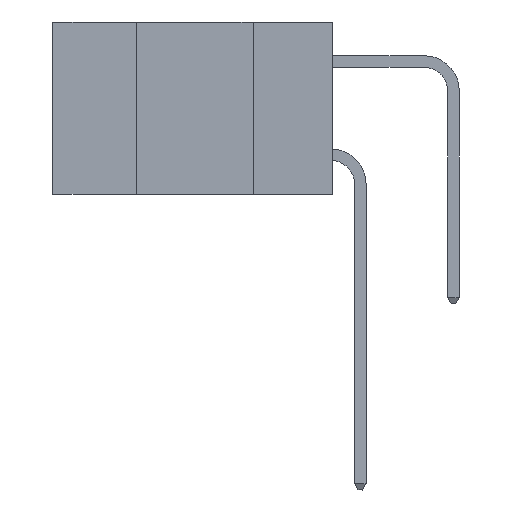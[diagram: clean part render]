
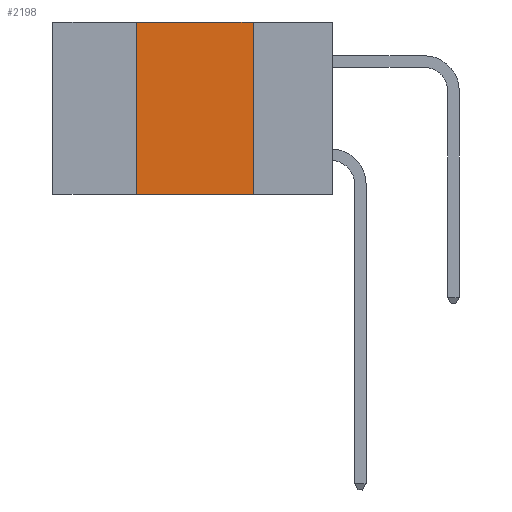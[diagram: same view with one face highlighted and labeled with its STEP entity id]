
A CAD part, left-side view. The second image highlights one B-rep face of the part: STEP entity #2198.
In plain terms, the highlighted planar face has unit normal (-1, 0, 0).
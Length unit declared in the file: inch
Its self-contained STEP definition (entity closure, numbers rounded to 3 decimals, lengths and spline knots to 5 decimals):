
#159 = CARTESIAN_POINT ( 'NONE',  ( 0., 0.17, 0. ) ) ;
#557 = VERTEX_POINT ( 'NONE', #20466 ) ;
#759 = VECTOR ( 'NONE', #14729, 39.37008 ) ;
#1258 = CARTESIAN_POINT ( 'NONE',  ( 0., 0.42, -0.37 ) ) ;
#1286 = LINE ( 'NONE', #1750, #15073 ) ;
#1750 = CARTESIAN_POINT ( 'NONE',  ( 0., 0.6, 0. ) ) ;
#1752 = LINE ( 'NONE', #10698, #31308 ) ;
#1899 = PLANE ( 'NONE',  #5361 ) ;
#1996 = VERTEX_POINT ( 'NONE', #25617 ) ;
#2198 = ADVANCED_FACE ( 'NONE', ( #20669 ), #1899, .F. ) ;
#3216 = DIRECTION ( 'NONE',  ( 0., -1., 0. ) ) ;
#5361 = AXIS2_PLACEMENT_3D ( 'NONE', #18979, #14195, #6666 ) ;
#6666 = DIRECTION ( 'NONE',  ( 0., 0., -1. ) ) ;
#7816 = EDGE_CURVE ( 'NONE', #21736, #1996, #13794, .T. ) ;
#10005 = DIRECTION ( 'NONE',  ( 0., 0., -1. ) ) ;
#10602 = ORIENTED_EDGE ( 'NONE', *, *, #11000, .F. ) ;
#10698 = CARTESIAN_POINT ( 'NONE',  ( 0., 0.6, -0.37 ) ) ;
#11000 = EDGE_CURVE ( 'NONE', #1996, #26828, #1286, .T. ) ;
#12233 = EDGE_LOOP ( 'NONE', ( #18242, #10602, #17671, #19631 ) ) ;
#12461 = LINE ( 'NONE', #159, #15150 ) ;
#12694 = EDGE_CURVE ( 'NONE', #21736, #557, #1752, .T. ) ;
#13794 = LINE ( 'NONE', #21779, #759 ) ;
#14195 = DIRECTION ( 'NONE',  ( 1., 0., 0. ) ) ;
#14729 = DIRECTION ( 'NONE',  ( 0., 0., 1. ) ) ;
#15073 = VECTOR ( 'NONE', #20963, 39.37008 ) ;
#15150 = VECTOR ( 'NONE', #10005, 39.37008 ) ;
#17671 = ORIENTED_EDGE ( 'NONE', *, *, #7816, .F. ) ;
#18242 = ORIENTED_EDGE ( 'NONE', *, *, #24576, .F. ) ;
#18979 = CARTESIAN_POINT ( 'NONE',  ( 0., 0.6, 0. ) ) ;
#19631 = ORIENTED_EDGE ( 'NONE', *, *, #12694, .T. ) ;
#20466 = CARTESIAN_POINT ( 'NONE',  ( 0., 0.17, -0.37 ) ) ;
#20669 = FACE_OUTER_BOUND ( 'NONE', #12233, .T. ) ;
#20963 = DIRECTION ( 'NONE',  ( 0., -1., 0. ) ) ;
#21736 = VERTEX_POINT ( 'NONE', #1258 ) ;
#21779 = CARTESIAN_POINT ( 'NONE',  ( 0., 0.42, 0. ) ) ;
#24576 = EDGE_CURVE ( 'NONE', #26828, #557, #12461, .T. ) ;
#25617 = CARTESIAN_POINT ( 'NONE',  ( 0., 0.42, 0. ) ) ;
#26828 = VERTEX_POINT ( 'NONE', #30565 ) ;
#30565 = CARTESIAN_POINT ( 'NONE',  ( 0., 0.17, 0. ) ) ;
#31308 = VECTOR ( 'NONE', #3216, 39.37008 ) ;
